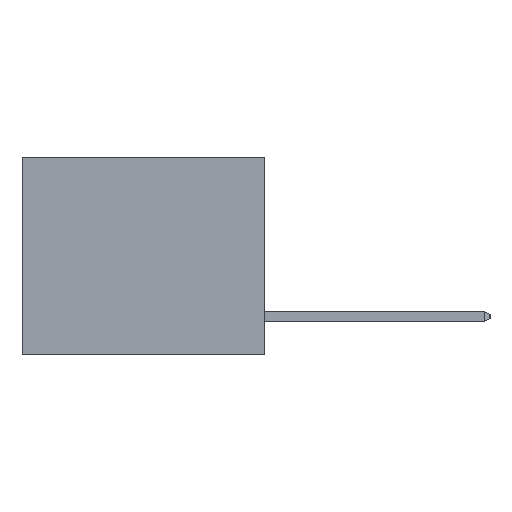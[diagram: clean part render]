
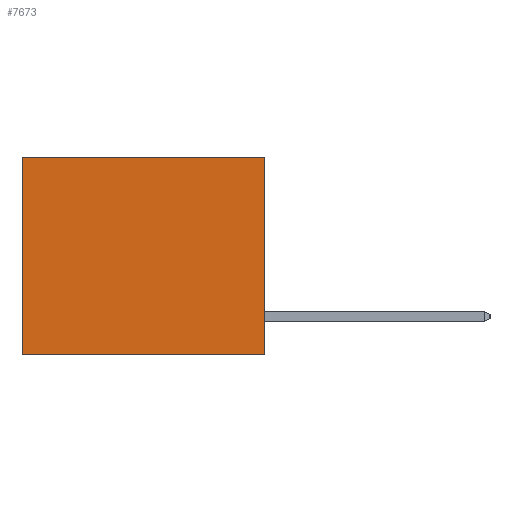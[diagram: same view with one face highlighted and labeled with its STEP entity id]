
A CAD part, left-side view. The second image highlights one B-rep face of the part: STEP entity #7673.
In plain terms, the highlighted planar face has unit normal (-1, 0, 0).
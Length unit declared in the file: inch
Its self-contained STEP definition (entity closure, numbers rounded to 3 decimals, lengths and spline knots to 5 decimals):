
#1017 = DIRECTION ( 'NONE',  ( 0., 0., -1. ) ) ;
#1138 = DIRECTION ( 'NONE',  ( 1., 0., 0. ) ) ;
#1171 = DIRECTION ( 'NONE',  ( 0., 0., -1. ) ) ;
#1173 = CARTESIAN_POINT ( 'NONE',  ( 0.3165, 0.6, 0. ) ) ;
#1538 = DIRECTION ( 'NONE',  ( 0., 1., 0. ) ) ;
#1943 = VERTEX_POINT ( 'NONE', #13921 ) ;
#2079 = EDGE_CURVE ( 'NONE', #10041, #1943, #3629, .T. ) ;
#2272 = CARTESIAN_POINT ( 'NONE',  ( 0.3165, 0., 0. ) ) ;
#2285 = VECTOR ( 'NONE', #11699, 39.37008 ) ;
#2437 = EDGE_LOOP ( 'NONE', ( #10096, #5813, #6206, #3949 ) ) ;
#2607 = EDGE_CURVE ( 'NONE', #1943, #7833, #11042, .T. ) ;
#2737 = EDGE_CURVE ( 'NONE', #10041, #9460, #11238, .T. ) ;
#3629 = LINE ( 'NONE', #4342, #2285 ) ;
#3949 = ORIENTED_EDGE ( 'NONE', *, *, #2737, .T. ) ;
#4342 = CARTESIAN_POINT ( 'NONE',  ( 0.3165, 0., -0.49 ) ) ;
#4796 = LINE ( 'NONE', #5883, #13427 ) ;
#5097 = CARTESIAN_POINT ( 'NONE',  ( 0.3165, 0.6, -0.49 ) ) ;
#5311 = VECTOR ( 'NONE', #8315, 39.37008 ) ;
#5813 = ORIENTED_EDGE ( 'NONE', *, *, #2607, .F. ) ;
#5883 = CARTESIAN_POINT ( 'NONE',  ( 0.3165, 0.6, -0.49 ) ) ;
#6206 = ORIENTED_EDGE ( 'NONE', *, *, #2079, .F. ) ;
#7497 = CARTESIAN_POINT ( 'NONE',  ( 0.3165, 0., -0.49 ) ) ;
#7673 = ADVANCED_FACE ( 'NONE', ( #12805 ), #14548, .F. ) ;
#7833 = VERTEX_POINT ( 'NONE', #5097 ) ;
#8315 = DIRECTION ( 'NONE',  ( 0., 1., 0. ) ) ;
#9460 = VERTEX_POINT ( 'NONE', #1173 ) ;
#10041 = VERTEX_POINT ( 'NONE', #12418 ) ;
#10096 = ORIENTED_EDGE ( 'NONE', *, *, #14334, .T. ) ;
#11042 = LINE ( 'NONE', #7497, #12604 ) ;
#11238 = LINE ( 'NONE', #2272, #5311 ) ;
#11699 = DIRECTION ( 'NONE',  ( 0., 0., -1. ) ) ;
#12418 = CARTESIAN_POINT ( 'NONE',  ( 0.3165, 0., 0. ) ) ;
#12604 = VECTOR ( 'NONE', #1538, 39.37008 ) ;
#12805 = FACE_OUTER_BOUND ( 'NONE', #2437, .T. ) ;
#13427 = VECTOR ( 'NONE', #1171, 39.37008 ) ;
#13921 = CARTESIAN_POINT ( 'NONE',  ( 0.3165, 0., -0.49 ) ) ;
#14334 = EDGE_CURVE ( 'NONE', #9460, #7833, #4796, .T. ) ;
#14338 = CARTESIAN_POINT ( 'NONE',  ( 0.3165, 0., -0.49 ) ) ;
#14363 = AXIS2_PLACEMENT_3D ( 'NONE', #14338, #1138, #1017 ) ;
#14548 = PLANE ( 'NONE',  #14363 ) ;
